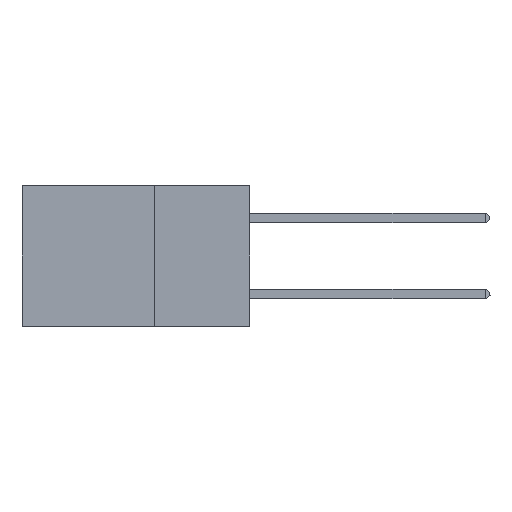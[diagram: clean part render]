
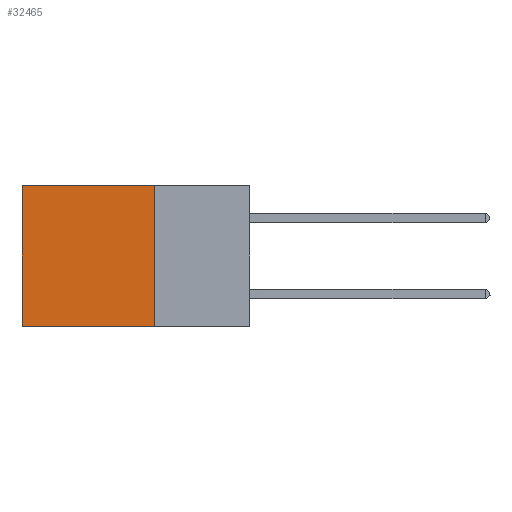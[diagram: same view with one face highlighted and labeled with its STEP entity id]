
A CAD part, left-side view. The second image highlights one B-rep face of the part: STEP entity #32465.
In plain terms, the highlighted planar face has unit normal (-1, 0, 0).
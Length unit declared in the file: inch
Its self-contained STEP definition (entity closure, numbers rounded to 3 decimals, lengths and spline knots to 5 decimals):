
#622 = VERTEX_POINT ( 'NONE', #17418 ) ;
#2566 = VECTOR ( 'NONE', #21800, 39.37008 ) ;
#3335 = ORIENTED_EDGE ( 'NONE', *, *, #44380, .F. ) ;
#6772 = CARTESIAN_POINT ( 'NONE',  ( 0.2875, 0.6, 0. ) ) ;
#7334 = PLANE ( 'NONE',  #32969 ) ;
#10826 = ORIENTED_EDGE ( 'NONE', *, *, #36268, .T. ) ;
#11172 = DIRECTION ( 'NONE',  ( 0., 0., -1. ) ) ;
#12279 = CARTESIAN_POINT ( 'NONE',  ( 0.2875, 0.25, 0. ) ) ;
#12499 = VECTOR ( 'NONE', #20051, 39.37008 ) ;
#12550 = CARTESIAN_POINT ( 'NONE',  ( 0.2875, 0.25, 0. ) ) ;
#13444 = ORIENTED_EDGE ( 'NONE', *, *, #45407, .T. ) ;
#16030 = VECTOR ( 'NONE', #40334, 39.37008 ) ;
#16645 = CARTESIAN_POINT ( 'NONE',  ( 0.2875, 0.6, -0.37 ) ) ;
#17253 = VERTEX_POINT ( 'NONE', #16645 ) ;
#17418 = CARTESIAN_POINT ( 'NONE',  ( 0.2875, 0.25, -0.37 ) ) ;
#17837 = EDGE_CURVE ( 'NONE', #18783, #622, #33199, .T. ) ;
#18783 = VERTEX_POINT ( 'NONE', #35387 ) ;
#20051 = DIRECTION ( 'NONE',  ( 0., 1., 0. ) ) ;
#21800 = DIRECTION ( 'NONE',  ( 0., 0., -1. ) ) ;
#22773 = LINE ( 'NONE', #6772, #2566 ) ;
#23285 = DIRECTION ( 'NONE',  ( 0., 0., -1. ) ) ;
#24045 = EDGE_LOOP ( 'NONE', ( #13444, #3335, #33866, #10826 ) ) ;
#28378 = FACE_OUTER_BOUND ( 'NONE', #24045, .T. ) ;
#30056 = VERTEX_POINT ( 'NONE', #43469 ) ;
#31723 = LINE ( 'NONE', #12550, #12499 ) ;
#32174 = VECTOR ( 'NONE', #23285, 39.37008 ) ;
#32465 = ADVANCED_FACE ( 'NONE', ( #28378 ), #7334, .F. ) ;
#32695 = CARTESIAN_POINT ( 'NONE',  ( 0.2875, 0.25, 0. ) ) ;
#32829 = DIRECTION ( 'NONE',  ( 1., 0., 0. ) ) ;
#32969 = AXIS2_PLACEMENT_3D ( 'NONE', #32695, #32829, #11172 ) ;
#33199 = LINE ( 'NONE', #12279, #32174 ) ;
#33866 = ORIENTED_EDGE ( 'NONE', *, *, #17837, .F. ) ;
#35387 = CARTESIAN_POINT ( 'NONE',  ( 0.2875, 0.25, 0. ) ) ;
#36268 = EDGE_CURVE ( 'NONE', #18783, #30056, #31723, .T. ) ;
#37023 = CARTESIAN_POINT ( 'NONE',  ( 0.2875, 0.25, -0.37 ) ) ;
#40334 = DIRECTION ( 'NONE',  ( 0., 1., 0. ) ) ;
#43469 = CARTESIAN_POINT ( 'NONE',  ( 0.2875, 0.6, 0. ) ) ;
#43790 = LINE ( 'NONE', #37023, #16030 ) ;
#44380 = EDGE_CURVE ( 'NONE', #622, #17253, #43790, .T. ) ;
#45407 = EDGE_CURVE ( 'NONE', #30056, #17253, #22773, .T. ) ;
